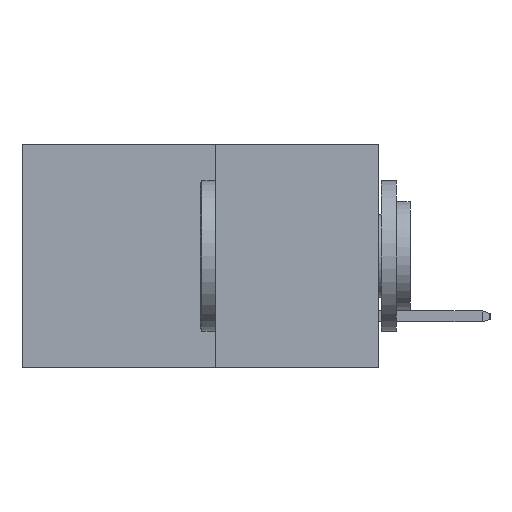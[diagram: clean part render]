
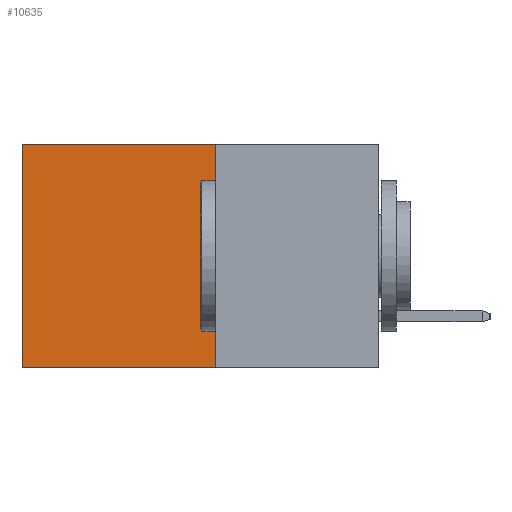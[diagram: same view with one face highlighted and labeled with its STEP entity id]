
A CAD part, left-side view. The second image highlights one B-rep face of the part: STEP entity #10635.
In plain terms, the highlighted planar face has unit normal (-1, 0, 0).
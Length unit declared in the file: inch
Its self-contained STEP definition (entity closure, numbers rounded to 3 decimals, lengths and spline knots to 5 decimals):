
#650 = CARTESIAN_POINT ( 'NONE',  ( 0.277, 0.27, -0.37 ) ) ;
#1258 = VERTEX_POINT ( 'NONE', #650 ) ;
#2259 = CARTESIAN_POINT ( 'NONE',  ( 0.277, 0.27, -0.37 ) ) ;
#2340 = VERTEX_POINT ( 'NONE', #9048 ) ;
#2555 = CARTESIAN_POINT ( 'NONE',  ( 0.277, 0.59, 0. ) ) ;
#3115 = DIRECTION ( 'NONE',  ( 0., 1., 0. ) ) ;
#3687 = PLANE ( 'NONE',  #11258 ) ;
#4374 = CARTESIAN_POINT ( 'NONE',  ( 0.277, 0.27, -0.37 ) ) ;
#4714 = EDGE_CURVE ( 'NONE', #1258, #2340, #10969, .T. ) ;
#5249 = VECTOR ( 'NONE', #6565, 39.37008 ) ;
#5912 = DIRECTION ( 'NONE',  ( 0., 0., -1. ) ) ;
#6565 = DIRECTION ( 'NONE',  ( 0., 0., -1. ) ) ;
#6784 = VECTOR ( 'NONE', #11581, 39.37008 ) ;
#7050 = ORIENTED_EDGE ( 'NONE', *, *, #7700, .T. ) ;
#7700 = EDGE_CURVE ( 'NONE', #9501, #8221, #9581, .T. ) ;
#7718 = CARTESIAN_POINT ( 'NONE',  ( 0.277, 0.59, -0.37 ) ) ;
#7904 = ORIENTED_EDGE ( 'NONE', *, *, #4714, .F. ) ;
#8028 = CARTESIAN_POINT ( 'NONE',  ( 0.277, 0.27, 0. ) ) ;
#8043 = LINE ( 'NONE', #4374, #5249 ) ;
#8221 = VERTEX_POINT ( 'NONE', #2555 ) ;
#8546 = VECTOR ( 'NONE', #3115, 39.37008 ) ;
#8836 = EDGE_LOOP ( 'NONE', ( #9404, #7904, #12357, #7050 ) ) ;
#9048 = CARTESIAN_POINT ( 'NONE',  ( 0.277, 0.59, -0.37 ) ) ;
#9357 = FACE_OUTER_BOUND ( 'NONE', #8836, .T. ) ;
#9404 = ORIENTED_EDGE ( 'NONE', *, *, #13144, .T. ) ;
#9501 = VERTEX_POINT ( 'NONE', #8028 ) ;
#9581 = LINE ( 'NONE', #13303, #6784 ) ;
#9880 = EDGE_CURVE ( 'NONE', #9501, #1258, #8043, .T. ) ;
#10288 = LINE ( 'NONE', #7718, #12703 ) ;
#10635 = ADVANCED_FACE ( 'NONE', ( #9357 ), #3687, .F. ) ;
#10888 = DIRECTION ( 'NONE',  ( 0., 0., -1. ) ) ;
#10969 = LINE ( 'NONE', #2259, #8546 ) ;
#11104 = CARTESIAN_POINT ( 'NONE',  ( 0.277, 0.27, -0.37 ) ) ;
#11258 = AXIS2_PLACEMENT_3D ( 'NONE', #11104, #12129, #5912 ) ;
#11581 = DIRECTION ( 'NONE',  ( 0., 1., 0. ) ) ;
#12129 = DIRECTION ( 'NONE',  ( 1., 0., 0. ) ) ;
#12357 = ORIENTED_EDGE ( 'NONE', *, *, #9880, .F. ) ;
#12703 = VECTOR ( 'NONE', #10888, 39.37008 ) ;
#13144 = EDGE_CURVE ( 'NONE', #8221, #2340, #10288, .T. ) ;
#13303 = CARTESIAN_POINT ( 'NONE',  ( 0.277, 0.27, 0. ) ) ;
